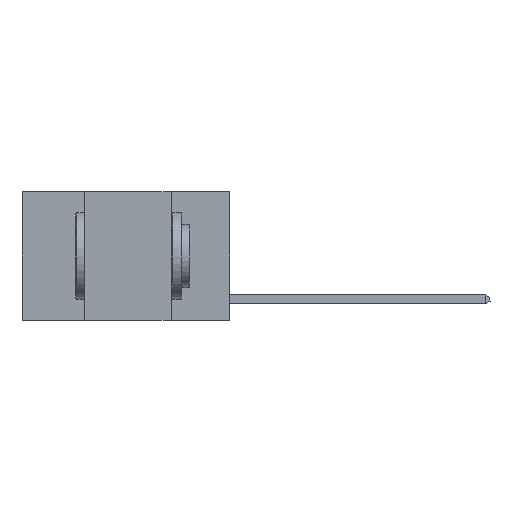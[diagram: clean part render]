
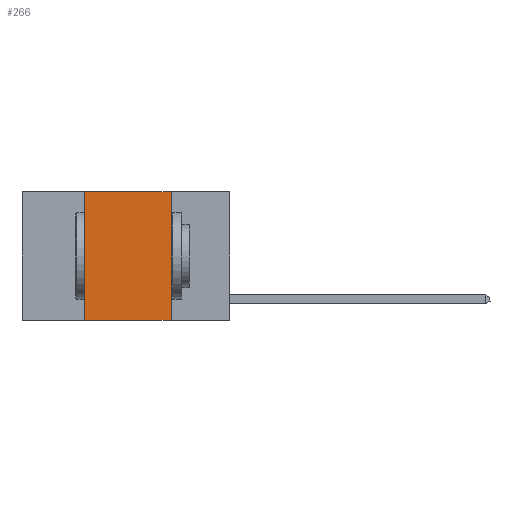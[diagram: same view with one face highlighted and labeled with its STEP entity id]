
A CAD part, left-side view. The second image highlights one B-rep face of the part: STEP entity #266.
In plain terms, the highlighted planar face has unit normal (-1, 0, 0).
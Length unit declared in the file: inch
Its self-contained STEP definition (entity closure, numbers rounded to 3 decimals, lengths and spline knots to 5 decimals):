
#266 = ADVANCED_FACE ( 'NONE', ( #11728 ), #5250, .F. ) ;
#383 = ORIENTED_EDGE ( 'NONE', *, *, #13346, .F. ) ;
#787 = VECTOR ( 'NONE', #9543, 39.37008 ) ;
#2155 = DIRECTION ( 'NONE',  ( 0., 0., 1. ) ) ;
#2243 = ORIENTED_EDGE ( 'NONE', *, *, #8647, .T. ) ;
#3049 = DIRECTION ( 'NONE',  ( 0., 0., -1. ) ) ;
#3298 = DIRECTION ( 'NONE',  ( 0., -1., 0. ) ) ;
#3348 = DIRECTION ( 'NONE',  ( 0., -1., 0. ) ) ;
#4782 = EDGE_CURVE ( 'NONE', #14068, #7631, #12707, .T. ) ;
#4792 = CARTESIAN_POINT ( 'NONE',  ( 0., 0.17, 0. ) ) ;
#5091 = VECTOR ( 'NONE', #3298, 39.37008 ) ;
#5250 = PLANE ( 'NONE',  #8294 ) ;
#6080 = ORIENTED_EDGE ( 'NONE', *, *, #12122, .F. ) ;
#6212 = CARTESIAN_POINT ( 'NONE',  ( 0., 0.6, 0. ) ) ;
#7335 = LINE ( 'NONE', #10378, #13955 ) ;
#7631 = VERTEX_POINT ( 'NONE', #12813 ) ;
#8256 = LINE ( 'NONE', #13988, #5091 ) ;
#8294 = AXIS2_PLACEMENT_3D ( 'NONE', #6212, #10278, #3049 ) ;
#8647 = EDGE_CURVE ( 'NONE', #13239, #13561, #8256, .T. ) ;
#9543 = DIRECTION ( 'NONE',  ( 0., 0., -1. ) ) ;
#10278 = DIRECTION ( 'NONE',  ( 1., 0., 0. ) ) ;
#10378 = CARTESIAN_POINT ( 'NONE',  ( 0., 0.42, 0. ) ) ;
#10395 = EDGE_LOOP ( 'NONE', ( #6080, #10990, #383, #2243 ) ) ;
#10418 = CARTESIAN_POINT ( 'NONE',  ( 0., 0.42, 0. ) ) ;
#10990 = ORIENTED_EDGE ( 'NONE', *, *, #4782, .F. ) ;
#11478 = CARTESIAN_POINT ( 'NONE',  ( 0., 0.6, 0. ) ) ;
#11626 = CARTESIAN_POINT ( 'NONE',  ( 0., 0.17, -0.37 ) ) ;
#11728 = FACE_OUTER_BOUND ( 'NONE', #10395, .T. ) ;
#12032 = LINE ( 'NONE', #4792, #787 ) ;
#12122 = EDGE_CURVE ( 'NONE', #7631, #13561, #12032, .T. ) ;
#12523 = VECTOR ( 'NONE', #3348, 39.37008 ) ;
#12707 = LINE ( 'NONE', #11478, #12523 ) ;
#12813 = CARTESIAN_POINT ( 'NONE',  ( 0., 0.17, 0. ) ) ;
#13239 = VERTEX_POINT ( 'NONE', #14101 ) ;
#13346 = EDGE_CURVE ( 'NONE', #13239, #14068, #7335, .T. ) ;
#13561 = VERTEX_POINT ( 'NONE', #11626 ) ;
#13955 = VECTOR ( 'NONE', #2155, 39.37008 ) ;
#13988 = CARTESIAN_POINT ( 'NONE',  ( 0., 0.6, -0.37 ) ) ;
#14068 = VERTEX_POINT ( 'NONE', #10418 ) ;
#14101 = CARTESIAN_POINT ( 'NONE',  ( 0., 0.42, -0.37 ) ) ;
